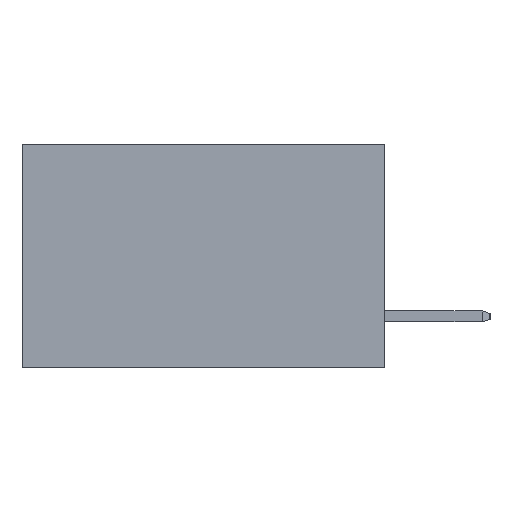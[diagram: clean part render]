
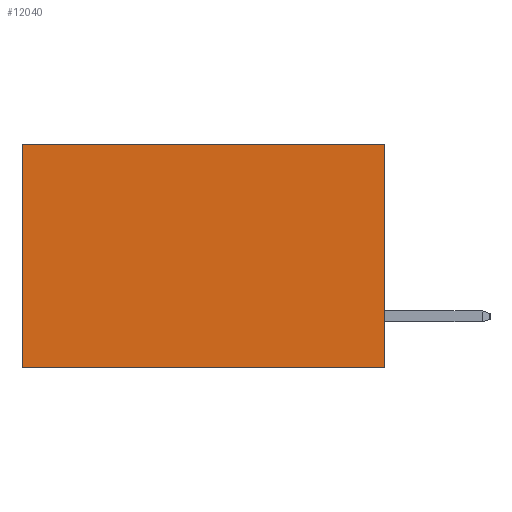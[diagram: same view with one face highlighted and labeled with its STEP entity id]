
A CAD part, left-side view. The second image highlights one B-rep face of the part: STEP entity #12040.
In plain terms, the highlighted planar face has unit normal (-1, 0, 0).
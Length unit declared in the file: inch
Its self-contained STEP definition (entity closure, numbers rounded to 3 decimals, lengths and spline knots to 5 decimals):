
#138 = ORIENTED_EDGE ( 'NONE', *, *, #2195, .F. ) ;
#402 = VERTEX_POINT ( 'NONE', #3660 ) ;
#628 = DIRECTION ( 'NONE',  ( 0., 0., -1. ) ) ;
#1023 = DIRECTION ( 'NONE',  ( 0., 0., -1. ) ) ;
#2031 = DIRECTION ( 'NONE',  ( 0., 1., 0. ) ) ;
#2195 = EDGE_CURVE ( 'NONE', #8597, #10030, #9709, .T. ) ;
#2387 = CARTESIAN_POINT ( 'NONE',  ( 0.298, 0.6, -0.37 ) ) ;
#2964 = ORIENTED_EDGE ( 'NONE', *, *, #6791, .T. ) ;
#3512 = ORIENTED_EDGE ( 'NONE', *, *, #7320, .F. ) ;
#3660 = CARTESIAN_POINT ( 'NONE',  ( 0.298, 0., 0. ) ) ;
#4032 = AXIS2_PLACEMENT_3D ( 'NONE', #12284, #6581, #628 ) ;
#5068 = DIRECTION ( 'NONE',  ( 0., 1., 0. ) ) ;
#5107 = VECTOR ( 'NONE', #1023, 39.37008 ) ;
#5407 = CARTESIAN_POINT ( 'NONE',  ( 0.298, 0., -0.37 ) ) ;
#5594 = PLANE ( 'NONE',  #4032 ) ;
#5626 = ORIENTED_EDGE ( 'NONE', *, *, #11172, .T. ) ;
#5750 = CARTESIAN_POINT ( 'NONE',  ( 0.298, 0., 0. ) ) ;
#6124 = DIRECTION ( 'NONE',  ( 0., 0., -1. ) ) ;
#6581 = DIRECTION ( 'NONE',  ( 1., 0., 0. ) ) ;
#6791 = EDGE_CURVE ( 'NONE', #402, #9668, #6934, .T. ) ;
#6934 = LINE ( 'NONE', #8719, #9150 ) ;
#7320 = EDGE_CURVE ( 'NONE', #402, #8597, #10207, .T. ) ;
#7923 = CARTESIAN_POINT ( 'NONE',  ( 0.298, 0., -0.37 ) ) ;
#8597 = VERTEX_POINT ( 'NONE', #7923 ) ;
#8628 = VECTOR ( 'NONE', #6124, 39.37008 ) ;
#8719 = CARTESIAN_POINT ( 'NONE',  ( 0.298, 0., 0. ) ) ;
#8852 = EDGE_LOOP ( 'NONE', ( #5626, #138, #3512, #2964 ) ) ;
#9150 = VECTOR ( 'NONE', #5068, 39.37008 ) ;
#9615 = CARTESIAN_POINT ( 'NONE',  ( 0.298, 0.6, 0. ) ) ;
#9668 = VERTEX_POINT ( 'NONE', #9615 ) ;
#9709 = LINE ( 'NONE', #5407, #11963 ) ;
#10030 = VERTEX_POINT ( 'NONE', #2387 ) ;
#10207 = LINE ( 'NONE', #5750, #5107 ) ;
#10840 = FACE_OUTER_BOUND ( 'NONE', #8852, .T. ) ;
#10865 = LINE ( 'NONE', #11848, #8628 ) ;
#11172 = EDGE_CURVE ( 'NONE', #9668, #10030, #10865, .T. ) ;
#11848 = CARTESIAN_POINT ( 'NONE',  ( 0.298, 0.6, 0. ) ) ;
#11963 = VECTOR ( 'NONE', #2031, 39.37008 ) ;
#12040 = ADVANCED_FACE ( 'NONE', ( #10840 ), #5594, .F. ) ;
#12284 = CARTESIAN_POINT ( 'NONE',  ( 0.298, 0., 0. ) ) ;
